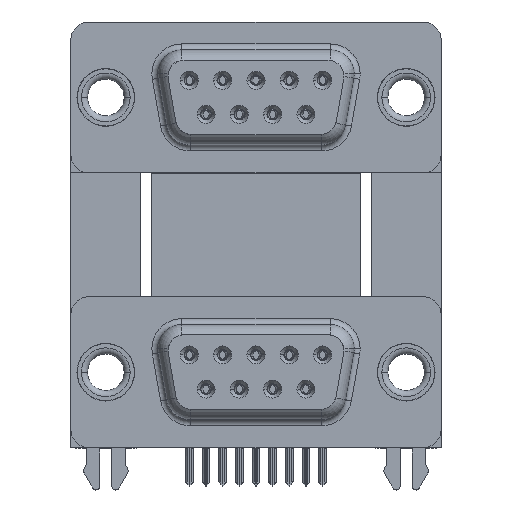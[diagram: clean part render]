
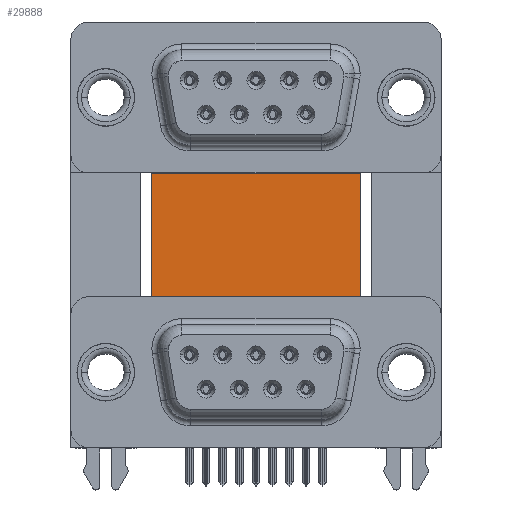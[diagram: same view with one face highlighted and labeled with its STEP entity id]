
A CAD part, top view. The second image highlights one B-rep face of the part: STEP entity #29888.
In plain terms, the highlighted planar face has unit normal (0, 0, 1).
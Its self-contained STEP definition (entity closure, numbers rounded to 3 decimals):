
#762 = DIRECTION ( 'NONE',  ( 0., 1., 0. ) ) ;
#910 = LINE ( 'NONE', #7417, #30728 ) ;
#1154 = VECTOR ( 'NONE', #30667, 1000. ) ;
#1589 = VECTOR ( 'NONE', #33007, 1000. ) ;
#2778 = LINE ( 'NONE', #18716, #17822 ) ;
#4609 = VERTEX_POINT ( 'NONE', #12756 ) ;
#4834 = CARTESIAN_POINT ( 'NONE',  ( 22.09, -4.635, -12. ) ) ;
#5072 = LINE ( 'NONE', #11342, #1154 ) ;
#5313 = CARTESIAN_POINT ( 'NONE',  ( 21.2, -0.735, -12. ) ) ;
#5331 = VECTOR ( 'NONE', #762, 1000. ) ;
#6231 = EDGE_CURVE ( 'NONE', #4609, #38582, #14343, .T. ) ;
#6615 = VECTOR ( 'NONE', #34307, 1000. ) ;
#6834 = ORIENTED_EDGE ( 'NONE', *, *, #28015, .T. ) ;
#7417 = CARTESIAN_POINT ( 'NONE',  ( 3.79, 16.585, -12. ) ) ;
#7664 = DIRECTION ( 'NONE',  ( 0., 0., -1. ) ) ;
#9625 = EDGE_CURVE ( 'NONE', #38582, #23876, #10554, .T. ) ;
#10554 = LINE ( 'NONE', #20588, #1589 ) ;
#10595 = CARTESIAN_POINT ( 'NONE',  ( 2.4, -4.635, -12. ) ) ;
#11205 = CARTESIAN_POINT ( 'NONE',  ( 3.79, -3.735, -12. ) ) ;
#11342 = CARTESIAN_POINT ( 'NONE',  ( 22.09, -4.635, -12. ) ) ;
#12598 = EDGE_CURVE ( 'NONE', #22747, #17059, #21968, .T. ) ;
#12756 = CARTESIAN_POINT ( 'NONE',  ( 2.9, -3.735, -12. ) ) ;
#14343 = LINE ( 'NONE', #11205, #6615 ) ;
#14985 = ORIENTED_EDGE ( 'NONE', *, *, #6231, .T. ) ;
#15130 = DIRECTION ( 'NONE',  ( 1., 0., 0. ) ) ;
#16033 = EDGE_CURVE ( 'NONE', #26922, #24765, #2778, .T. ) ;
#16305 = CARTESIAN_POINT ( 'NONE',  ( 3.79, 16.585, -12. ) ) ;
#16808 = CARTESIAN_POINT ( 'NONE',  ( 22.09, -3.735, -12. ) ) ;
#17059 = VERTEX_POINT ( 'NONE', #5313 ) ;
#17149 = EDGE_CURVE ( 'NONE', #25368, #22747, #31936, .T. ) ;
#17822 = VECTOR ( 'NONE', #15130, 1000. ) ;
#18203 = ORIENTED_EDGE ( 'NONE', *, *, #25774, .T. ) ;
#18291 = DIRECTION ( 'NONE',  ( 1., 0., 0. ) ) ;
#18716 = CARTESIAN_POINT ( 'NONE',  ( 2.9, -4.635, -12. ) ) ;
#19024 = ORIENTED_EDGE ( 'NONE', *, *, #19608, .T. ) ;
#19530 = VERTEX_POINT ( 'NONE', #22541 ) ;
#19608 = EDGE_CURVE ( 'NONE', #19530, #26922, #30434, .T. ) ;
#19627 = CARTESIAN_POINT ( 'NONE',  ( 2.9, -4.635, -12. ) ) ;
#19813 = CARTESIAN_POINT ( 'NONE',  ( 3.79, 16.585, -12. ) ) ;
#19907 = EDGE_LOOP ( 'NONE', ( #14985, #35361, #18203, #39650, #30690, #20499, #6834, #19024, #37350, #37380 ) ) ;
#20499 = ORIENTED_EDGE ( 'NONE', *, *, #17149, .F. ) ;
#20588 = CARTESIAN_POINT ( 'NONE',  ( 22.09, -3.735, -12. ) ) ;
#20628 = AXIS2_PLACEMENT_3D ( 'NONE', #19813, #7664, #23586 ) ;
#21318 = CARTESIAN_POINT ( 'NONE',  ( 22.59, -4.635, -12. ) ) ;
#21749 = CARTESIAN_POINT ( 'NONE',  ( 21.2, 16.585, -12. ) ) ;
#21968 = LINE ( 'NONE', #21749, #36156 ) ;
#22380 = DIRECTION ( 'NONE',  ( 0., -1., 0. ) ) ;
#22396 = VECTOR ( 'NONE', #24322, 1000. ) ;
#22541 = CARTESIAN_POINT ( 'NONE',  ( 3.79, -0.735, -12. ) ) ;
#22747 = VERTEX_POINT ( 'NONE', #36114 ) ;
#23345 = DIRECTION ( 'NONE',  ( 0., -1., 0. ) ) ;
#23586 = DIRECTION ( 'NONE',  ( -1., 0., 0. ) ) ;
#23591 = CARTESIAN_POINT ( 'NONE',  ( 2.9, -3.735, -12. ) ) ;
#23876 = VERTEX_POINT ( 'NONE', #4834 ) ;
#23898 = VECTOR ( 'NONE', #18291, 1000. ) ;
#24322 = DIRECTION ( 'NONE',  ( -0.336, -0.942, 0. ) ) ;
#24600 = EDGE_CURVE ( 'NONE', #27516, #17059, #34154, .T. ) ;
#24765 = VERTEX_POINT ( 'NONE', #19627 ) ;
#25368 = VERTEX_POINT ( 'NONE', #16305 ) ;
#25774 = EDGE_CURVE ( 'NONE', #23876, #27516, #5072, .T. ) ;
#26129 = LINE ( 'NONE', #23591, #5331 ) ;
#26922 = VERTEX_POINT ( 'NONE', #10595 ) ;
#27516 = VERTEX_POINT ( 'NONE', #38760 ) ;
#27826 = DIRECTION ( 'NONE',  ( -0.336, 0.942, 0. ) ) ;
#28015 = EDGE_CURVE ( 'NONE', #25368, #19530, #910, .T. ) ;
#29672 = PLANE ( 'NONE',  #20628 ) ;
#29888 = ADVANCED_FACE ( 'NONE', ( #32851 ), #29672, .F. ) ;
#30434 = LINE ( 'NONE', #33598, #22396 ) ;
#30667 = DIRECTION ( 'NONE',  ( 1., 0., 0. ) ) ;
#30690 = ORIENTED_EDGE ( 'NONE', *, *, #12598, .F. ) ;
#30728 = VECTOR ( 'NONE', #23345, 1000. ) ;
#31014 = EDGE_CURVE ( 'NONE', #24765, #4609, #26129, .T. ) ;
#31936 = LINE ( 'NONE', #41002, #23898 ) ;
#32851 = FACE_OUTER_BOUND ( 'NONE', #19907, .T. ) ;
#33007 = DIRECTION ( 'NONE',  ( 0., -1., 0. ) ) ;
#33598 = CARTESIAN_POINT ( 'NONE',  ( 2.4, -4.635, -12. ) ) ;
#34154 = LINE ( 'NONE', #21318, #38109 ) ;
#34307 = DIRECTION ( 'NONE',  ( 1., 0., 0. ) ) ;
#35361 = ORIENTED_EDGE ( 'NONE', *, *, #9625, .T. ) ;
#36114 = CARTESIAN_POINT ( 'NONE',  ( 21.2, 16.585, -12. ) ) ;
#36156 = VECTOR ( 'NONE', #22380, 1000. ) ;
#37350 = ORIENTED_EDGE ( 'NONE', *, *, #16033, .T. ) ;
#37380 = ORIENTED_EDGE ( 'NONE', *, *, #31014, .T. ) ;
#38109 = VECTOR ( 'NONE', #27826, 1000. ) ;
#38582 = VERTEX_POINT ( 'NONE', #16808 ) ;
#38760 = CARTESIAN_POINT ( 'NONE',  ( 22.59, -4.635, -12. ) ) ;
#39650 = ORIENTED_EDGE ( 'NONE', *, *, #24600, .T. ) ;
#41002 = CARTESIAN_POINT ( 'NONE',  ( 3.79, 16.585, -12. ) ) ;
